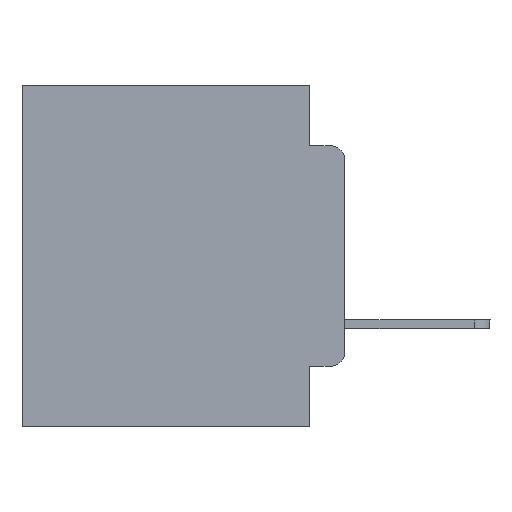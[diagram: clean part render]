
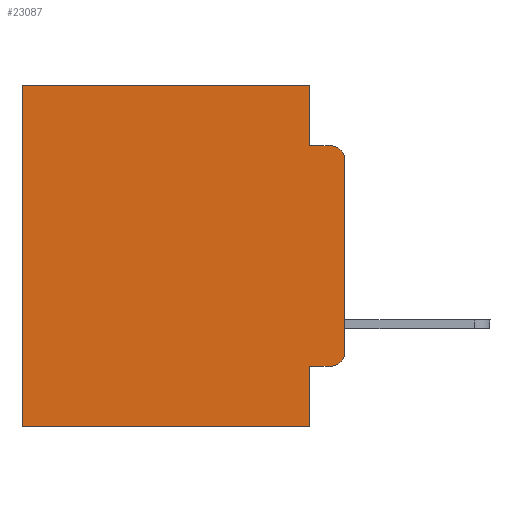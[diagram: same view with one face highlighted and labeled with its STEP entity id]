
A CAD part, left-side view. The second image highlights one B-rep face of the part: STEP entity #23087.
In plain terms, the highlighted planar face has unit normal (-1, 0, 0).
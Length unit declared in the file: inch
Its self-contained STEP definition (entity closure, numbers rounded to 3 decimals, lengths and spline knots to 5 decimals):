
#730 = CARTESIAN_POINT ( 'NONE',  ( 0.298, 0., 0. ) ) ;
#901 = LINE ( 'NONE', #8438, #13823 ) ;
#1009 = CIRCLE ( 'NONE', #10031, 0.02 ) ;
#1100 = LINE ( 'NONE', #730, #21313 ) ;
#1178 = LINE ( 'NONE', #3048, #18336 ) ;
#1386 = VERTEX_POINT ( 'NONE', #5370 ) ;
#1584 = EDGE_CURVE ( 'NONE', #6216, #6689, #7920, .T. ) ;
#1986 = EDGE_LOOP ( 'NONE', ( #23442, #9798, #4619, #21030, #7273, #20728, #21481, #7584, #20150, #3764 ) ) ;
#2087 = CARTESIAN_POINT ( 'NONE',  ( 0.298, 0.02, -0.4115 ) ) ;
#2150 = CARTESIAN_POINT ( 'NONE',  ( 0.298, 0.051, -0.0885 ) ) ;
#3048 = CARTESIAN_POINT ( 'NONE',  ( 0.298, 0.051, 0. ) ) ;
#3218 = DIRECTION ( 'NONE',  ( 0., 0., -1. ) ) ;
#3439 = LINE ( 'NONE', #11089, #21158 ) ;
#3593 = VERTEX_POINT ( 'NONE', #15156 ) ;
#3683 = EDGE_CURVE ( 'NONE', #3593, #18520, #1009, .T. ) ;
#3762 = LINE ( 'NONE', #3863, #13583 ) ;
#3764 = ORIENTED_EDGE ( 'NONE', *, *, #6652, .T. ) ;
#3863 = CARTESIAN_POINT ( 'NONE',  ( 0.298, 0.051, 0. ) ) ;
#4243 = VERTEX_POINT ( 'NONE', #8559 ) ;
#4602 = VECTOR ( 'NONE', #24797, 39.37008 ) ;
#4616 = DIRECTION ( 'NONE',  ( 0., 1., 0. ) ) ;
#4619 = ORIENTED_EDGE ( 'NONE', *, *, #5994, .F. ) ;
#4820 = VECTOR ( 'NONE', #22827, 39.37008 ) ;
#5370 = CARTESIAN_POINT ( 'NONE',  ( 0.298, 0., -0.3915 ) ) ;
#5520 = VERTEX_POINT ( 'NONE', #16506 ) ;
#5642 = VERTEX_POINT ( 'NONE', #20828 ) ;
#5669 = AXIS2_PLACEMENT_3D ( 'NONE', #7802, #21359, #23246 ) ;
#5994 = EDGE_CURVE ( 'NONE', #16340, #18520, #3439, .T. ) ;
#6216 = VERTEX_POINT ( 'NONE', #9799 ) ;
#6241 = EDGE_CURVE ( 'NONE', #5642, #6689, #901, .T. ) ;
#6585 = CARTESIAN_POINT ( 'NONE',  ( 0.298, 0.02, -0.0885 ) ) ;
#6652 = EDGE_CURVE ( 'NONE', #8416, #1386, #24178, .T. ) ;
#6689 = VERTEX_POINT ( 'NONE', #13380 ) ;
#7273 = ORIENTED_EDGE ( 'NONE', *, *, #8058, .T. ) ;
#7584 = ORIENTED_EDGE ( 'NONE', *, *, #15965, .F. ) ;
#7802 = CARTESIAN_POINT ( 'NONE',  ( 0.298, 0.02, -0.3915 ) ) ;
#7920 = LINE ( 'NONE', #20927, #12495 ) ;
#8058 = EDGE_CURVE ( 'NONE', #5520, #5642, #1100, .T. ) ;
#8416 = VERTEX_POINT ( 'NONE', #2087 ) ;
#8438 = CARTESIAN_POINT ( 'NONE',  ( 0.298, 0.473, 0. ) ) ;
#8527 = LINE ( 'NONE', #19069, #4820 ) ;
#8559 = CARTESIAN_POINT ( 'NONE',  ( 0.298, 0.051, -0.4115 ) ) ;
#9054 = DIRECTION ( 'NONE',  ( 0., -1., 0. ) ) ;
#9798 = ORIENTED_EDGE ( 'NONE', *, *, #3683, .T. ) ;
#9799 = CARTESIAN_POINT ( 'NONE',  ( 0.298, 0.051, -0.5 ) ) ;
#10031 = AXIS2_PLACEMENT_3D ( 'NONE', #14776, #17073, #3218 ) ;
#10156 = CARTESIAN_POINT ( 'NONE',  ( 0.298, 0., 0. ) ) ;
#10380 = DIRECTION ( 'NONE',  ( 0., 0., -1. ) ) ;
#10970 = FACE_OUTER_BOUND ( 'NONE', #1986, .T. ) ;
#11089 = CARTESIAN_POINT ( 'NONE',  ( 0.298, 0.051, -0.0885 ) ) ;
#12495 = VECTOR ( 'NONE', #13268, 39.37008 ) ;
#13174 = CARTESIAN_POINT ( 'NONE',  ( 0.298, 0., 0. ) ) ;
#13268 = DIRECTION ( 'NONE',  ( 0., 1., 0. ) ) ;
#13380 = CARTESIAN_POINT ( 'NONE',  ( 0.298, 0.473, -0.5 ) ) ;
#13583 = VECTOR ( 'NONE', #13967, 39.37008 ) ;
#13758 = EDGE_CURVE ( 'NONE', #5520, #16340, #3762, .T. ) ;
#13823 = VECTOR ( 'NONE', #10380, 39.37008 ) ;
#13967 = DIRECTION ( 'NONE',  ( 0., 0., -1. ) ) ;
#14776 = CARTESIAN_POINT ( 'NONE',  ( 0.298, 0.02, -0.1085 ) ) ;
#15156 = CARTESIAN_POINT ( 'NONE',  ( 0.298, 0., -0.1085 ) ) ;
#15451 = AXIS2_PLACEMENT_3D ( 'NONE', #10156, #23824, #16069 ) ;
#15518 = EDGE_CURVE ( 'NONE', #3593, #1386, #24805, .T. ) ;
#15965 = EDGE_CURVE ( 'NONE', #4243, #6216, #1178, .T. ) ;
#16069 = DIRECTION ( 'NONE',  ( 0., 0., -1. ) ) ;
#16340 = VERTEX_POINT ( 'NONE', #2150 ) ;
#16506 = CARTESIAN_POINT ( 'NONE',  ( 0.298, 0.051, 0. ) ) ;
#16571 = DIRECTION ( 'NONE',  ( 0., 0., -1. ) ) ;
#16774 = EDGE_CURVE ( 'NONE', #4243, #8416, #8527, .T. ) ;
#17073 = DIRECTION ( 'NONE',  ( -1., 0., 0. ) ) ;
#18336 = VECTOR ( 'NONE', #16571, 39.37008 ) ;
#18520 = VERTEX_POINT ( 'NONE', #6585 ) ;
#19069 = CARTESIAN_POINT ( 'NONE',  ( 0.298, 0.051, -0.4115 ) ) ;
#19875 = PLANE ( 'NONE',  #15451 ) ;
#20150 = ORIENTED_EDGE ( 'NONE', *, *, #16774, .T. ) ;
#20728 = ORIENTED_EDGE ( 'NONE', *, *, #6241, .T. ) ;
#20828 = CARTESIAN_POINT ( 'NONE',  ( 0.298, 0.473, 0. ) ) ;
#20927 = CARTESIAN_POINT ( 'NONE',  ( 0.298, 0., -0.5 ) ) ;
#21030 = ORIENTED_EDGE ( 'NONE', *, *, #13758, .F. ) ;
#21158 = VECTOR ( 'NONE', #9054, 39.37008 ) ;
#21313 = VECTOR ( 'NONE', #4616, 39.37008 ) ;
#21359 = DIRECTION ( 'NONE',  ( -1., 0., 0. ) ) ;
#21481 = ORIENTED_EDGE ( 'NONE', *, *, #1584, .F. ) ;
#22827 = DIRECTION ( 'NONE',  ( 0., -1., 0. ) ) ;
#23087 = ADVANCED_FACE ( 'NONE', ( #10970 ), #19875, .F. ) ;
#23246 = DIRECTION ( 'NONE',  ( 0., 0., -1. ) ) ;
#23442 = ORIENTED_EDGE ( 'NONE', *, *, #15518, .F. ) ;
#23824 = DIRECTION ( 'NONE',  ( 1., 0., 0. ) ) ;
#24178 = CIRCLE ( 'NONE', #5669, 0.02 ) ;
#24797 = DIRECTION ( 'NONE',  ( 0., 0., -1. ) ) ;
#24805 = LINE ( 'NONE', #13174, #4602 ) ;
